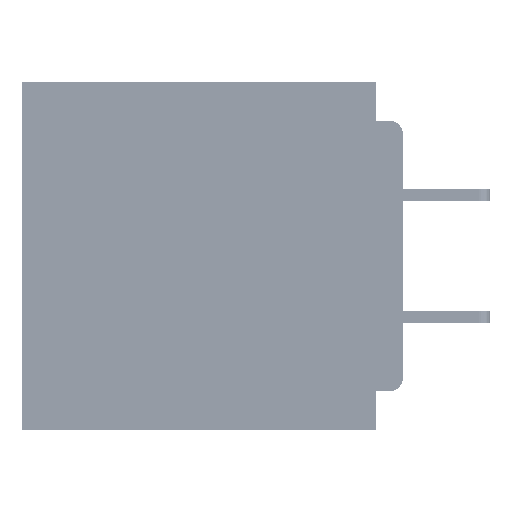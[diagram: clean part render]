
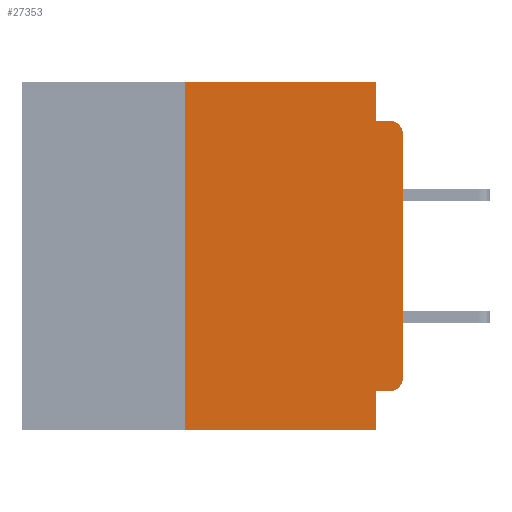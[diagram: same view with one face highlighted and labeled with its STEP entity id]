
A CAD part, left-side view. The second image highlights one B-rep face of the part: STEP entity #27353.
In plain terms, the highlighted planar face has unit normal (-1, 0, 0).
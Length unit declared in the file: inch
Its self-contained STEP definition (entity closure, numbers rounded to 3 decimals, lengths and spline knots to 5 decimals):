
#2116 = CARTESIAN_POINT ( 'NONE',  ( 0., 0.25, -0.4 ) ) ;
#2334 = DIRECTION ( 'NONE',  ( -1., 0., 0. ) ) ;
#2498 = DIRECTION ( 'NONE',  ( 0., 0., -1. ) ) ;
#2654 = ORIENTED_EDGE ( 'NONE', *, *, #57334, .F. ) ;
#3146 = AXIS2_PLACEMENT_3D ( 'NONE', #34900, #2334, #40365 ) ;
#5124 = DIRECTION ( 'NONE',  ( 0., -1., 0. ) ) ;
#5728 = ORIENTED_EDGE ( 'NONE', *, *, #53038, .F. ) ;
#6275 = VERTEX_POINT ( 'NONE', #63704 ) ;
#6441 = DIRECTION ( 'NONE',  ( 0., 0., -1. ) ) ;
#6679 = VERTEX_POINT ( 'NONE', #24846 ) ;
#7772 = CARTESIAN_POINT ( 'NONE',  ( 0., 0.031, -0.4 ) ) ;
#9476 = VERTEX_POINT ( 'NONE', #55583 ) ;
#10953 = ORIENTED_EDGE ( 'NONE', *, *, #53872, .F. ) ;
#11400 = LINE ( 'NONE', #63447, #67215 ) ;
#11666 = CARTESIAN_POINT ( 'NONE',  ( 0., 0.015, -0.045 ) ) ;
#11748 = CARTESIAN_POINT ( 'NONE',  ( 0., 0., -0.045 ) ) ;
#11801 = CARTESIAN_POINT ( 'NONE',  ( 0., 0.437, -0.4 ) ) ;
#15473 = CARTESIAN_POINT ( 'NONE',  ( 0., 0., -0.06 ) ) ;
#15941 = ORIENTED_EDGE ( 'NONE', *, *, #32416, .F. ) ;
#17369 = LINE ( 'NONE', #67407, #58907 ) ;
#20593 = EDGE_LOOP ( 'NONE', ( #46923, #55136, #2654, #39346, #68971, #5728, #43485, #10953, #15941, #38883 ) ) ;
#20737 = EDGE_CURVE ( 'NONE', #32171, #57972, #42077, .T. ) ;
#21708 = CARTESIAN_POINT ( 'NONE',  ( 0., 0.25, 0. ) ) ;
#23552 = EDGE_CURVE ( 'NONE', #34245, #6679, #23821, .T. ) ;
#23651 = LINE ( 'NONE', #49802, #65124 ) ;
#23821 = LINE ( 'NONE', #59179, #33139 ) ;
#24846 = CARTESIAN_POINT ( 'NONE',  ( 0., 0.031, 0. ) ) ;
#25125 = CARTESIAN_POINT ( 'NONE',  ( 0., 0.031, -0.355 ) ) ;
#25720 = EDGE_CURVE ( 'NONE', #9476, #50130, #59586, .T. ) ;
#25725 = CARTESIAN_POINT ( 'NONE',  ( 0., 0.015, -0.34 ) ) ;
#27353 = ADVANCED_FACE ( 'NONE', ( #66052 ), #65891, .F. ) ;
#28010 = EDGE_CURVE ( 'NONE', #50130, #32171, #23651, .T. ) ;
#28134 = DIRECTION ( 'NONE',  ( 0., -1., 0. ) ) ;
#28256 = LINE ( 'NONE', #11748, #57069 ) ;
#29212 = VERTEX_POINT ( 'NONE', #34222 ) ;
#30760 = VERTEX_POINT ( 'NONE', #25125 ) ;
#31166 = DIRECTION ( 'NONE',  ( 0., 0., -1. ) ) ;
#32171 = VERTEX_POINT ( 'NONE', #15473 ) ;
#32416 = EDGE_CURVE ( 'NONE', #9476, #30760, #41921, .T. ) ;
#33139 = VECTOR ( 'NONE', #5124, 39.37008 ) ;
#33429 = DIRECTION ( 'NONE',  ( 0., 0., 1. ) ) ;
#33510 = CARTESIAN_POINT ( 'NONE',  ( 0., 0.437, 0. ) ) ;
#34222 = CARTESIAN_POINT ( 'NONE',  ( 0., 0.25, -0.4 ) ) ;
#34245 = VERTEX_POINT ( 'NONE', #21708 ) ;
#34900 = CARTESIAN_POINT ( 'NONE',  ( 0., 0.015, -0.06 ) ) ;
#38137 = AXIS2_PLACEMENT_3D ( 'NONE', #33510, #38990, #6441 ) ;
#38515 = DIRECTION ( 'NONE',  ( 0., 1., 0. ) ) ;
#38883 = ORIENTED_EDGE ( 'NONE', *, *, #25720, .T. ) ;
#38990 = DIRECTION ( 'NONE',  ( 1., 0., 0. ) ) ;
#39346 = ORIENTED_EDGE ( 'NONE', *, *, #56418, .F. ) ;
#40365 = DIRECTION ( 'NONE',  ( 0., 0., -1. ) ) ;
#41921 = LINE ( 'NONE', #49200, #52924 ) ;
#42077 = CIRCLE ( 'NONE', #3146, 0.015 ) ;
#43485 = ORIENTED_EDGE ( 'NONE', *, *, #56840, .T. ) ;
#46144 = LINE ( 'NONE', #11801, #62181 ) ;
#46923 = ORIENTED_EDGE ( 'NONE', *, *, #28010, .T. ) ;
#47424 = DIRECTION ( 'NONE',  ( 0., 0., -1. ) ) ;
#47694 = VERTEX_POINT ( 'NONE', #7772 ) ;
#48000 = VECTOR ( 'NONE', #51083, 39.37008 ) ;
#49200 = CARTESIAN_POINT ( 'NONE',  ( 0., 0., -0.355 ) ) ;
#49680 = DIRECTION ( 'NONE',  ( 0., -1., 0. ) ) ;
#49802 = CARTESIAN_POINT ( 'NONE',  ( 0., 0., 0. ) ) ;
#50130 = VERTEX_POINT ( 'NONE', #53992 ) ;
#51083 = DIRECTION ( 'NONE',  ( 0., 0., 1. ) ) ;
#52924 = VECTOR ( 'NONE', #38515, 39.37008 ) ;
#53038 = EDGE_CURVE ( 'NONE', #29212, #34245, #64014, .T. ) ;
#53872 = EDGE_CURVE ( 'NONE', #30760, #47694, #11400, .T. ) ;
#53992 = CARTESIAN_POINT ( 'NONE',  ( 0., 0., -0.34 ) ) ;
#55136 = ORIENTED_EDGE ( 'NONE', *, *, #20737, .T. ) ;
#55583 = CARTESIAN_POINT ( 'NONE',  ( 0., 0.015, -0.355 ) ) ;
#56418 = EDGE_CURVE ( 'NONE', #6679, #6275, #17369, .T. ) ;
#56840 = EDGE_CURVE ( 'NONE', #29212, #47694, #46144, .T. ) ;
#57069 = VECTOR ( 'NONE', #49680, 39.37008 ) ;
#57334 = EDGE_CURVE ( 'NONE', #6275, #57972, #28256, .T. ) ;
#57972 = VERTEX_POINT ( 'NONE', #11666 ) ;
#58907 = VECTOR ( 'NONE', #2498, 39.37008 ) ;
#59179 = CARTESIAN_POINT ( 'NONE',  ( 0., 0.437, 0. ) ) ;
#59586 = CIRCLE ( 'NONE', #68698, 0.015 ) ;
#62181 = VECTOR ( 'NONE', #28134, 39.37008 ) ;
#63447 = CARTESIAN_POINT ( 'NONE',  ( 0., 0.031, -0.4 ) ) ;
#63571 = DIRECTION ( 'NONE',  ( -1., 0., 0. ) ) ;
#63704 = CARTESIAN_POINT ( 'NONE',  ( 0., 0.031, -0.045 ) ) ;
#64014 = LINE ( 'NONE', #2116, #48000 ) ;
#65124 = VECTOR ( 'NONE', #33429, 39.37008 ) ;
#65891 = PLANE ( 'NONE',  #38137 ) ;
#66052 = FACE_OUTER_BOUND ( 'NONE', #20593, .T. ) ;
#67215 = VECTOR ( 'NONE', #47424, 39.37008 ) ;
#67407 = CARTESIAN_POINT ( 'NONE',  ( 0., 0.031, 0. ) ) ;
#68698 = AXIS2_PLACEMENT_3D ( 'NONE', #25725, #63571, #31166 ) ;
#68971 = ORIENTED_EDGE ( 'NONE', *, *, #23552, .F. ) ;
